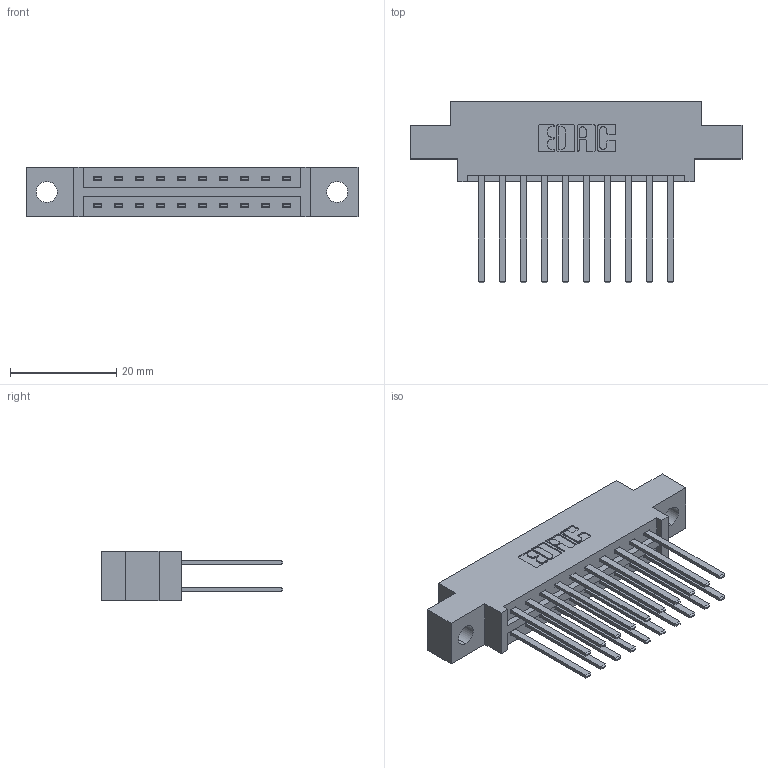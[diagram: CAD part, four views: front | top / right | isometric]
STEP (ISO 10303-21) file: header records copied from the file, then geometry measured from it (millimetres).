
FILE_DESCRIPTION (( 'STEP AP203' ), '1' );
FILE_NAME ('337-020-544-804.STEP', '2019-10-10T19:30:46', ( '' ), ( '' ), 'SwSTEP 2.0', 'SolidWorks 2016', '' );
FILE_SCHEMA (( 'CONFIG_CONTROL_DESIGN' ));
Length unit declared in the file: inch
Products named in the file (3): 345-292-001_345-293-144; 337-020-544-804; 337 Part_0.170 Offset - 0.156 Dia-TH
Assembly tree (21 placements, depth 2):
  337-020-544-804
    337 Part_0.170 Offset - 0.156 Dia-TH
    345-292-001_345-293-144  x20
Bounding box: 62.64 x 34.3 x 9.4 mm (x, y, z)
Volume: 6250.2 mm3; surface area: 7576.1 mm2
Topology: 21 solids, 21 shells, 1078 faces, 3183 edges, 2094 vertices
Faces by surface type: plane 754, cylinder 324
Entity records: 11843 total; most frequent: CARTESIAN_POINT 2022, ORIENTED_EDGE 1958, DIRECTION 1775, EDGE_CURVE 979, LINE 855, VECTOR 855, VERTEX_POINT 650, AXIS2_PLACEMENT_3D 460
